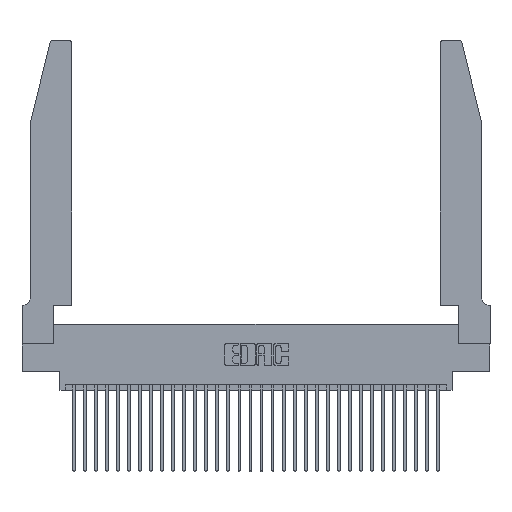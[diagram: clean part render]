
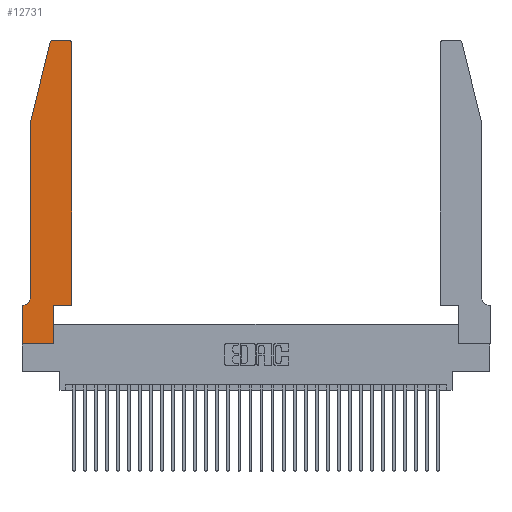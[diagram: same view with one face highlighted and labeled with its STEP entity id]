
A CAD part, top view. The second image highlights one B-rep face of the part: STEP entity #12731.
In plain terms, the highlighted planar face has unit normal (0, 0, 1).
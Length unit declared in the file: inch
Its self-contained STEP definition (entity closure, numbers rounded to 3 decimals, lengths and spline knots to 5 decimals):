
#41 = DIRECTION ( 'NONE',  ( 0., -1., 0. ) ) ;
#291 = CARTESIAN_POINT ( 'NONE',  ( 0., 0.35, 0.37 ) ) ;
#416 = ORIENTED_EDGE ( 'NONE', *, *, #16679, .T. ) ;
#765 = ORIENTED_EDGE ( 'NONE', *, *, #8805, .T. ) ;
#995 = VERTEX_POINT ( 'NONE', #27373 ) ;
#1052 = ORIENTED_EDGE ( 'NONE', *, *, #7404, .T. ) ;
#1209 = DIRECTION ( 'NONE',  ( 1., 0., 0. ) ) ;
#1500 = ORIENTED_EDGE ( 'NONE', *, *, #12469, .T. ) ;
#1607 = DIRECTION ( 'NONE',  ( 1., 0., 0. ) ) ;
#1886 = VECTOR ( 'NONE', #8560, 39.37008 ) ;
#2561 = LINE ( 'NONE', #21194, #21247 ) ;
#2708 = VERTEX_POINT ( 'NONE', #3126 ) ;
#2932 = DIRECTION ( 'NONE',  ( 0., 0., 1. ) ) ;
#3126 = CARTESIAN_POINT ( 'NONE',  ( 0.0055, 0.35, 0.37 ) ) ;
#3737 = CARTESIAN_POINT ( 'NONE',  ( 0.0055, 0.42, 0.37 ) ) ;
#4377 = VECTOR ( 'NONE', #12406, 39.37008 ) ;
#4640 = VECTOR ( 'NONE', #22121, 39.37008 ) ;
#4949 = DIRECTION ( 'NONE',  ( 0., -1., 0. ) ) ;
#5011 = VERTEX_POINT ( 'NONE', #19774 ) ;
#5746 = EDGE_CURVE ( 'NONE', #5011, #19763, #6753, .T. ) ;
#5893 = EDGE_CURVE ( 'NONE', #18902, #15531, #8760, .T. ) ;
#6041 = CARTESIAN_POINT ( 'NONE',  ( 0.25487, 2.72718, 0.37 ) ) ;
#6194 = DIRECTION ( 'NONE',  ( 0., 0., 1. ) ) ;
#6329 = DIRECTION ( 'NONE',  ( -1., 0., 0. ) ) ;
#6753 = CIRCLE ( 'NONE', #24483, 0.03 ) ;
#7275 = ORIENTED_EDGE ( 'NONE', *, *, #27867, .T. ) ;
#7404 = EDGE_CURVE ( 'NONE', #15458, #5011, #32157, .T. ) ;
#8400 = LINE ( 'NONE', #31445, #21022 ) ;
#8432 = VERTEX_POINT ( 'NONE', #291 ) ;
#8560 = DIRECTION ( 'NONE',  ( 1., 0., 0. ) ) ;
#8760 = LINE ( 'NONE', #18641, #1886 ) ;
#8805 = EDGE_CURVE ( 'NONE', #15531, #25057, #22785, .T. ) ;
#8880 = ORIENTED_EDGE ( 'NONE', *, *, #21035, .T. ) ;
#9155 = ORIENTED_EDGE ( 'NONE', *, *, #25982, .T. ) ;
#10089 = EDGE_CURVE ( 'NONE', #8432, #18902, #17285, .T. ) ;
#10223 = VECTOR ( 'NONE', #32041, 39.37008 ) ;
#10943 = CARTESIAN_POINT ( 'NONE',  ( 0.2865, 0., 0.37 ) ) ;
#11855 = VERTEX_POINT ( 'NONE', #20594 ) ;
#12406 = DIRECTION ( 'NONE',  ( 0., 1., 0. ) ) ;
#12469 = EDGE_CURVE ( 'NONE', #15062, #995, #26882, .T. ) ;
#12609 = CARTESIAN_POINT ( 'NONE',  ( 0., 0., 0.37 ) ) ;
#12731 = ADVANCED_FACE ( 'NONE', ( #27628 ), #14460, .T. ) ;
#12921 = CARTESIAN_POINT ( 'NONE',  ( 0.0755, 2., 0.37 ) ) ;
#13675 = ORIENTED_EDGE ( 'NONE', *, *, #5893, .T. ) ;
#14460 = PLANE ( 'NONE',  #22090 ) ;
#14671 = CARTESIAN_POINT ( 'NONE',  ( 0.2865, 0.35, 0.37 ) ) ;
#14944 = CARTESIAN_POINT ( 'NONE',  ( 0.4505, 0.35, 0.37 ) ) ;
#14958 = AXIS2_PLACEMENT_3D ( 'NONE', #21363, #6194, #23850 ) ;
#15062 = VERTEX_POINT ( 'NONE', #23336 ) ;
#15176 = ORIENTED_EDGE ( 'NONE', *, *, #22682, .T. ) ;
#15371 = CARTESIAN_POINT ( 'NONE',  ( 0.0755, 2., 0.37 ) ) ;
#15458 = VERTEX_POINT ( 'NONE', #20604 ) ;
#15531 = VERTEX_POINT ( 'NONE', #10943 ) ;
#16492 = VECTOR ( 'NONE', #4949, 39.37008 ) ;
#16679 = EDGE_CURVE ( 'NONE', #25057, #11855, #8400, .T. ) ;
#16950 = DIRECTION ( 'NONE',  ( 0., 0., 1. ) ) ;
#17285 = LINE ( 'NONE', #12609, #16492 ) ;
#17960 = ORIENTED_EDGE ( 'NONE', *, *, #10089, .T. ) ;
#18223 = CARTESIAN_POINT ( 'NONE',  ( 0.284, 2.72, 0.37 ) ) ;
#18641 = CARTESIAN_POINT ( 'NONE',  ( 0., 0., 0.37 ) ) ;
#18902 = VERTEX_POINT ( 'NONE', #25798 ) ;
#19640 = CARTESIAN_POINT ( 'NONE',  ( 0.2605, 2.75, 0.37 ) ) ;
#19763 = VERTEX_POINT ( 'NONE', #6041 ) ;
#19774 = CARTESIAN_POINT ( 'NONE',  ( 0.284, 2.75, 0.37 ) ) ;
#20305 = CARTESIAN_POINT ( 'NONE',  ( 0.4505, 2.72, 0.37 ) ) ;
#20396 = VECTOR ( 'NONE', #30388, 39.37008 ) ;
#20594 = CARTESIAN_POINT ( 'NONE',  ( 0.4505, 0.35, 0.37 ) ) ;
#20604 = CARTESIAN_POINT ( 'NONE',  ( 0.4205, 2.75, 0.37 ) ) ;
#20728 = DIRECTION ( 'NONE',  ( 1., 0., 0. ) ) ;
#21022 = VECTOR ( 'NONE', #1209, 39.37008 ) ;
#21035 = EDGE_CURVE ( 'NONE', #30278, #15458, #23107, .T. ) ;
#21171 = LINE ( 'NONE', #15371, #20396 ) ;
#21194 = CARTESIAN_POINT ( 'NONE',  ( 0.0755, 0.35, 0.37 ) ) ;
#21247 = VECTOR ( 'NONE', #26295, 39.37008 ) ;
#21363 = CARTESIAN_POINT ( 'NONE',  ( 0.4205, 2.72, 0.37 ) ) ;
#21485 = DIRECTION ( 'NONE',  ( 0., 0., -1. ) ) ;
#21661 = EDGE_LOOP ( 'NONE', ( #1052, #22135, #9155, #1500, #15176, #30410, #17960, #13675, #765, #416, #7275, #8880 ) ) ;
#22090 = AXIS2_PLACEMENT_3D ( 'NONE', #31826, #16950, #1607 ) ;
#22121 = DIRECTION ( 'NONE',  ( -1., 0., 0. ) ) ;
#22135 = ORIENTED_EDGE ( 'NONE', *, *, #5746, .T. ) ;
#22486 = CIRCLE ( 'NONE', #32454, 0.07 ) ;
#22682 = EDGE_CURVE ( 'NONE', #995, #2708, #22486, .T. ) ;
#22785 = LINE ( 'NONE', #14671, #10223 ) ;
#23107 = CIRCLE ( 'NONE', #14958, 0.03 ) ;
#23336 = CARTESIAN_POINT ( 'NONE',  ( 0.0755, 2., 0.37 ) ) ;
#23850 = DIRECTION ( 'NONE',  ( 1., 0., 0. ) ) ;
#23912 = EDGE_CURVE ( 'NONE', #2708, #8432, #2561, .T. ) ;
#24483 = AXIS2_PLACEMENT_3D ( 'NONE', #18223, #2932, #20728 ) ;
#25057 = VERTEX_POINT ( 'NONE', #30814 ) ;
#25798 = CARTESIAN_POINT ( 'NONE',  ( 0., 0., 0.37 ) ) ;
#25982 = EDGE_CURVE ( 'NONE', #19763, #15062, #21171, .T. ) ;
#26295 = DIRECTION ( 'NONE',  ( -1., 0., 0. ) ) ;
#26882 = LINE ( 'NONE', #12921, #27660 ) ;
#27373 = CARTESIAN_POINT ( 'NONE',  ( 0.0755, 0.42, 0.37 ) ) ;
#27628 = FACE_OUTER_BOUND ( 'NONE', #21661, .T. ) ;
#27660 = VECTOR ( 'NONE', #41, 39.37008 ) ;
#27867 = EDGE_CURVE ( 'NONE', #11855, #30278, #31136, .T. ) ;
#30278 = VERTEX_POINT ( 'NONE', #20305 ) ;
#30388 = DIRECTION ( 'NONE',  ( -0.239, -0.971, 0. ) ) ;
#30410 = ORIENTED_EDGE ( 'NONE', *, *, #23912, .T. ) ;
#30814 = CARTESIAN_POINT ( 'NONE',  ( 0.2865, 0.35, 0.37 ) ) ;
#31136 = LINE ( 'NONE', #14944, #4377 ) ;
#31445 = CARTESIAN_POINT ( 'NONE',  ( 0.4505, 0.35, 0.37 ) ) ;
#31826 = CARTESIAN_POINT ( 'NONE',  ( 0., 0.35, 0.37 ) ) ;
#32041 = DIRECTION ( 'NONE',  ( 0., 1., 0. ) ) ;
#32157 = LINE ( 'NONE', #19640, #4640 ) ;
#32454 = AXIS2_PLACEMENT_3D ( 'NONE', #3737, #21485, #6329 ) ;
